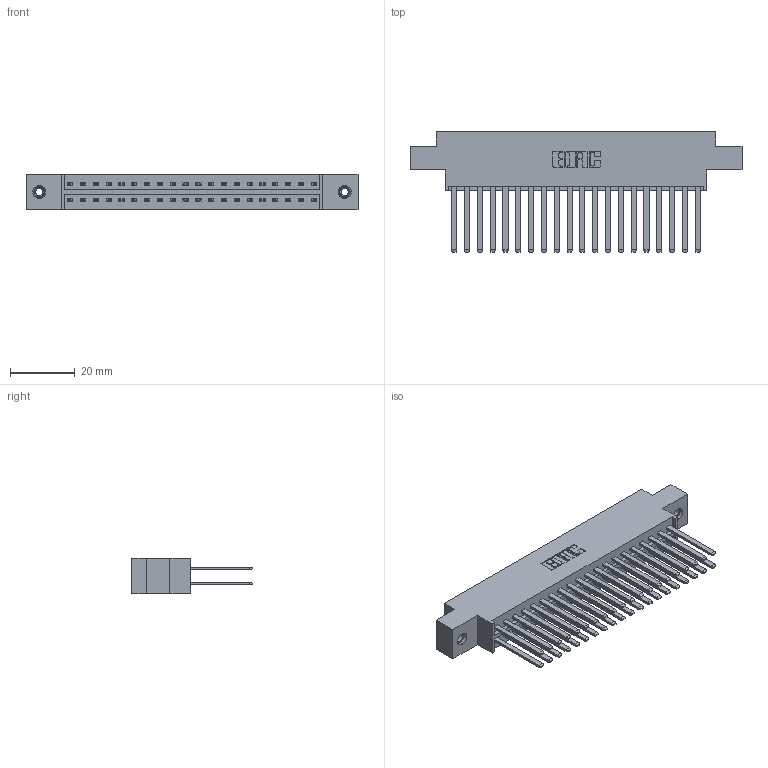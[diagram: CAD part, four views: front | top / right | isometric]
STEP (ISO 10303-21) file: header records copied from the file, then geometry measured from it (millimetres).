
FILE_DESCRIPTION (( 'STEP AP203' ), '1' );
FILE_NAME ('336-040-541-808.STEP', '2020-08-07T23:23:55', ( '' ), ( '' ), 'SwSTEP 2.0', 'SolidWorks 2020', '' );
FILE_SCHEMA (( 'CONFIG_CONTROL_DESIGN' ));
Length unit declared in the file: inch
Products named in the file (4): 336-290-001_336-290-541; 345-250-001_345-250-003-102; 336-040-541-808; 336 Part_Offset - .156 Dia - TI
Assembly tree (43 placements, depth 2):
  336-040-541-808
    336 Part_Offset - .156 Dia - TI
    336-290-001_336-290-541  x40
    345-250-001_345-250-003-102  x2
Bounding box: 102.64 x 37.34 x 11.1 mm (x, y, z)
Volume: 15123.1 mm3; surface area: 18988.9 mm2
Topology: 43 solids, 43 shells, 1858 faces, 5539 edges, 3658 vertices
Faces by surface type: plane 1146, cylinder 696, cone 12, torus 4
Entity records: 19389 total; most frequent: CARTESIAN_POINT 3348, ORIENTED_EDGE 3178, DIRECTION 2823, EDGE_CURVE 1589, VECTOR 1437, LINE 1437, VERTEX_POINT 1054, AXIS2_PLACEMENT_3D 693
